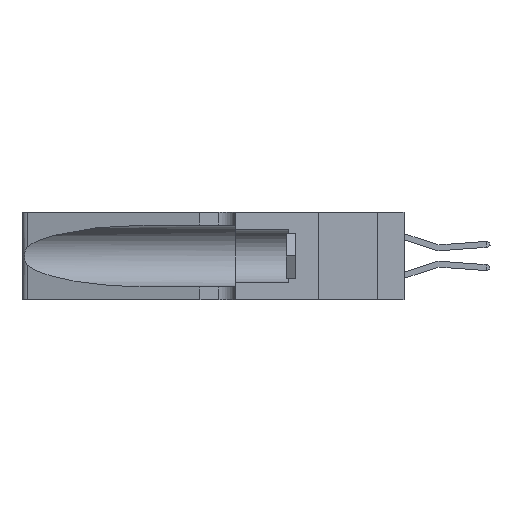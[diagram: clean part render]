
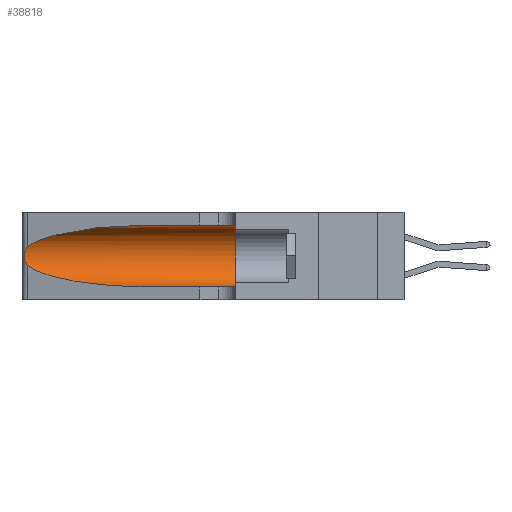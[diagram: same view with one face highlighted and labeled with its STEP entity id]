
A CAD part, left-side view. The second image highlights one B-rep face of the part: STEP entity #38818.
In plain terms, the highlighted cylindrical face has radius 3.308 mm (diameter 6.617 mm), a partial arc.
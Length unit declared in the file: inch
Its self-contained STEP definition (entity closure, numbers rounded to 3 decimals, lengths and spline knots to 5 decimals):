
#859 = CARTESIAN_POINT ( 'NONE',  ( 0.25487, 1.22718, 0.14631 ) ) ;
#1004 = CARTESIAN_POINT ( 'NONE',  ( 0.1305, 0.72297, 0.05475 ) ) ;
#1934 = CARTESIAN_POINT ( 'NONE',  ( 0.1305, 1.61858, 0.185 ) ) ;
#2134 = CARTESIAN_POINT ( 'NONE',  ( 0.25487, 1.22718, 0.22369 ) ) ;
#2282 = CARTESIAN_POINT ( 'NONE',  ( 0.26075, 1.23896, 0.19203 ) ) ;
#3622 = EDGE_CURVE ( 'NONE', #20210, #4421, #9934, .T. ) ;
#3996 = VECTOR ( 'NONE', #33093, 39.37008 ) ;
#4182 = CARTESIAN_POINT ( 'NONE',  ( 0.1305, 1.61858, 0.05475 ) ) ;
#4421 = VERTEX_POINT ( 'NONE', #24280 ) ;
#5289 = DIRECTION ( 'NONE',  ( 0., -1., 0. ) ) ;
#5621 = CARTESIAN_POINT ( 'NONE',  ( 0.26017, 1.23833, 0.17102 ) ) ;
#8679 = AXIS2_PLACEMENT_3D ( 'NONE', #1934, #5289, #14871 ) ;
#8885 = CARTESIAN_POINT ( 'NONE',  ( 0.25789, 1.23486, 0.15765 ) ) ;
#9934 = LINE ( 'NONE', #4182, #24869 ) ;
#11092 = EDGE_LOOP ( 'NONE', ( #38555, #28579, #20227, #33491, #16464, #29775 ) ) ;
#11971 = CARTESIAN_POINT ( 'NONE',  ( 0.25555, 1.22994, 0.2215 ) ) ;
#12110 = CARTESIAN_POINT ( 'NONE',  ( 0.25555, 1.22993, 0.14849 ) ) ;
#13455 = DIRECTION ( 'NONE',  ( 0., 1., 0. ) ) ;
#13533 = AXIS2_PLACEMENT_3D ( 'NONE', #32320, #13455, #35480 ) ;
#14155 = B_SPLINE_CURVE_WITH_KNOTS ( 'NONE', 3,
 ( #2134, #11971, #37204, #18414, #40336, #21577, #2282, #24754, #5621, #27889, #8885, #31023, #12110, #34176 ),
 .UNSPECIFIED., .F., .F.,
 ( 4, 2, 2, 2, 2, 2, 4 ),
 ( 0., 0.00027, 0.00053, 0.00107, 0.0016, 0.00187, 0.00214 ),
 .UNSPECIFIED. ) ;
#14829 = CARTESIAN_POINT ( 'NONE',  ( 0.25487, 1.22718, 0.14631 ) ) ;
#14871 = DIRECTION ( 'NONE',  ( 0., 0., -1. ) ) ;
#16464 = ORIENTED_EDGE ( 'NONE', *, *, #39537, .F. ) ;
#17261 = EDGE_CURVE ( 'NONE', #31111, #30329, #29390, .T. ) ;
#17913 = CARTESIAN_POINT ( 'NONE',  ( 0.18966, 0.96281, 0.31525 ) ) ;
#18173 = CARTESIAN_POINT ( 'NONE',  ( 0.1305, 0.72297, 0.05475 ) ) ;
#18414 = CARTESIAN_POINT ( 'NONE',  ( 0.25787, 1.23484, 0.2124 ) ) ;
#19206 = FACE_OUTER_BOUND ( 'NONE', #11092, .T. ) ;
#20210 = VERTEX_POINT ( 'NONE', #18173 ) ;
#20227 = ORIENTED_EDGE ( 'NONE', *, *, #24767, .T. ) ;
#20368 = CARTESIAN_POINT ( 'NONE',  ( 0.18966, 0.96281, 0.05475 ) ) ;
#21228 = CARTESIAN_POINT ( 'NONE',  ( 0.25487, 1.22718, 0.22369 ) ) ;
#21577 = CARTESIAN_POINT ( 'NONE',  ( 0.26018, 1.23835, 0.19895 ) ) ;
#23505 = CARTESIAN_POINT ( 'NONE',  ( 0.1305, 0.35, 0.31525 ) ) ;
#24280 = CARTESIAN_POINT ( 'NONE',  ( 0.1305, 0.35, 0.05475 ) ) ;
#24754 = CARTESIAN_POINT ( 'NONE',  ( 0.26075, 1.23896, 0.178 ) ) ;
#24767 = EDGE_CURVE ( 'NONE', #34804, #20210, #28799, .T. ) ;
#24869 = VECTOR ( 'NONE', #32798, 39.37008 ) ;
#25392 = VERTEX_POINT ( 'NONE', #29601 ) ;
#26534 = CARTESIAN_POINT ( 'NONE',  ( 0.2373, 1.15595, 0.08982 ) ) ;
#27889 = CARTESIAN_POINT ( 'NONE',  ( 0.25856, 1.23593, 0.16098 ) ) ;
#28579 = ORIENTED_EDGE ( 'NONE', *, *, #29967, .T. ) ;
#28799 =( BOUNDED_CURVE ( )  B_SPLINE_CURVE ( 3, ( #859, #26534, #20368, #1004 ),
 .UNSPECIFIED., .F., .T. ) 
 B_SPLINE_CURVE_WITH_KNOTS ( ( 4, 4 ),
 ( 3.44316, 4.71239 ),
 .UNSPECIFIED. ) 
 CURVE ( )  GEOMETRIC_REPRESENTATION_ITEM ( )  RATIONAL_B_SPLINE_CURVE ( ( 1., 0.87, 0.87, 1. ) ) 
 REPRESENTATION_ITEM ( '' )  );
#29390 = LINE ( 'NONE', #29922, #3996 ) ;
#29601 = CARTESIAN_POINT ( 'NONE',  ( 0.25487, 1.22718, 0.22369 ) ) ;
#29775 = ORIENTED_EDGE ( 'NONE', *, *, #17261, .F. ) ;
#29922 = CARTESIAN_POINT ( 'NONE',  ( 0.1305, 1.61858, 0.31525 ) ) ;
#29967 = EDGE_CURVE ( 'NONE', #25392, #34804, #14155, .T. ) ;
#30329 = VERTEX_POINT ( 'NONE', #23505 ) ;
#31023 = CARTESIAN_POINT ( 'NONE',  ( 0.25639, 1.23186, 0.15144 ) ) ;
#31111 = VERTEX_POINT ( 'NONE', #39444 ) ;
#31380 = CIRCLE ( 'NONE', #13533, 0.13025 ) ;
#32320 = CARTESIAN_POINT ( 'NONE',  ( 0.1305, 0.35, 0.185 ) ) ;
#32798 = DIRECTION ( 'NONE',  ( 0., -1., 0. ) ) ;
#33069 =( BOUNDED_CURVE ( )  B_SPLINE_CURVE ( 3, ( #33661, #17913, #39973, #21228 ),
 .UNSPECIFIED., .F., .F. ) 
 B_SPLINE_CURVE_WITH_KNOTS ( ( 4, 4 ),
 ( 1.5708, 2.84003 ),
 .UNSPECIFIED. ) 
 CURVE ( )  GEOMETRIC_REPRESENTATION_ITEM ( )  RATIONAL_B_SPLINE_CURVE ( ( 1., 0.87, 0.87, 1. ) ) 
 REPRESENTATION_ITEM ( '' )  );
#33093 = DIRECTION ( 'NONE',  ( 0., -1., 0. ) ) ;
#33491 = ORIENTED_EDGE ( 'NONE', *, *, #3622, .T. ) ;
#33661 = CARTESIAN_POINT ( 'NONE',  ( 0.1305, 0.72297, 0.31525 ) ) ;
#33896 = CYLINDRICAL_SURFACE ( 'NONE', #8679, 0.13025 ) ;
#34176 = CARTESIAN_POINT ( 'NONE',  ( 0.25487, 1.22718, 0.14631 ) ) ;
#34801 = EDGE_CURVE ( 'NONE', #31111, #25392, #33069, .T. ) ;
#34804 = VERTEX_POINT ( 'NONE', #14829 ) ;
#35480 = DIRECTION ( 'NONE',  ( 0., 0., 1. ) ) ;
#37204 = CARTESIAN_POINT ( 'NONE',  ( 0.25639, 1.23184, 0.21858 ) ) ;
#38555 = ORIENTED_EDGE ( 'NONE', *, *, #34801, .T. ) ;
#38818 = ADVANCED_FACE ( 'NONE', ( #19206 ), #33896, .F. ) ;
#39444 = CARTESIAN_POINT ( 'NONE',  ( 0.1305, 0.72297, 0.31525 ) ) ;
#39537 = EDGE_CURVE ( 'NONE', #30329, #4421, #31380, .T. ) ;
#39973 = CARTESIAN_POINT ( 'NONE',  ( 0.2373, 1.15595, 0.28018 ) ) ;
#40336 = CARTESIAN_POINT ( 'NONE',  ( 0.25854, 1.2359, 0.20912 ) ) ;
